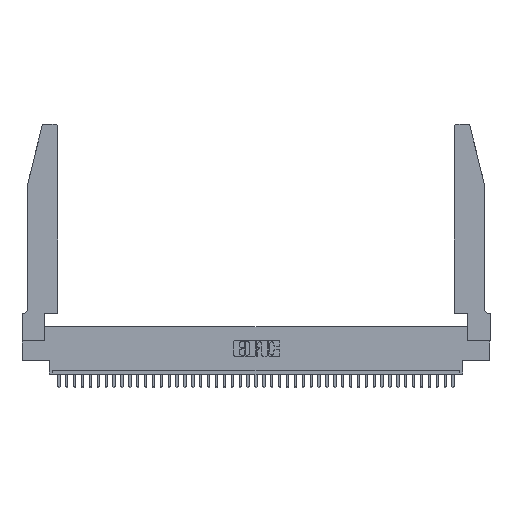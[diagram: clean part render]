
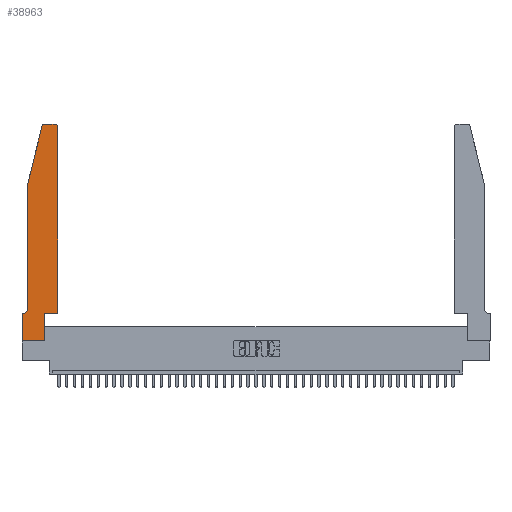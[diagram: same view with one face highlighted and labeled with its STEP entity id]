
A CAD part, top view. The second image highlights one B-rep face of the part: STEP entity #38963.
In plain terms, the highlighted planar face has unit normal (0, 0, 1).
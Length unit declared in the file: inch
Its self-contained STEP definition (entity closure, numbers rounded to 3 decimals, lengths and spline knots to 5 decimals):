
#378 = VECTOR ( 'NONE', #20610, 39.37008 ) ;
#417 = DIRECTION ( 'NONE',  ( 0., 0., 1. ) ) ;
#780 = VERTEX_POINT ( 'NONE', #36501 ) ;
#1311 = VERTEX_POINT ( 'NONE', #11483 ) ;
#1314 = VERTEX_POINT ( 'NONE', #11922 ) ;
#1644 = ORIENTED_EDGE ( 'NONE', *, *, #15194, .T. ) ;
#1787 = AXIS2_PLACEMENT_3D ( 'NONE', #8677, #15035, #21431 ) ;
#1841 = ORIENTED_EDGE ( 'NONE', *, *, #27327, .T. ) ;
#2714 = VECTOR ( 'NONE', #11933, 39.37008 ) ;
#3234 = VECTOR ( 'NONE', #31210, 39.37008 ) ;
#3577 = CIRCLE ( 'NONE', #1787, 0.07 ) ;
#3644 = LINE ( 'NONE', #36861, #30088 ) ;
#3887 = DIRECTION ( 'NONE',  ( 0., 0., 1. ) ) ;
#4013 = ORIENTED_EDGE ( 'NONE', *, *, #22150, .T. ) ;
#4426 = VERTEX_POINT ( 'NONE', #34378 ) ;
#4610 = DIRECTION ( 'NONE',  ( 0., -1., 0. ) ) ;
#5189 = CARTESIAN_POINT ( 'NONE',  ( 0.284, 2.72, 0.37 ) ) ;
#7242 = VERTEX_POINT ( 'NONE', #28314 ) ;
#7512 = CARTESIAN_POINT ( 'NONE',  ( 0.0755, 2., 0.37 ) ) ;
#8570 = ORIENTED_EDGE ( 'NONE', *, *, #21283, .T. ) ;
#8677 = CARTESIAN_POINT ( 'NONE',  ( 0.0055, 0.42, 0.37 ) ) ;
#8825 = VERTEX_POINT ( 'NONE', #28804 ) ;
#8885 = LINE ( 'NONE', #33943, #2714 ) ;
#9082 = AXIS2_PLACEMENT_3D ( 'NONE', #39704, #3887, #14320 ) ;
#9258 = DIRECTION ( 'NONE',  ( 0., 1., 0. ) ) ;
#10153 = VERTEX_POINT ( 'NONE', #36741 ) ;
#10204 = EDGE_LOOP ( 'NONE', ( #28763, #8570, #1841, #1644, #36367, #24538, #15567, #11738, #4013, #31337, #11991, #17164 ) ) ;
#10351 = AXIS2_PLACEMENT_3D ( 'NONE', #5189, #15029, #18297 ) ;
#10630 = VECTOR ( 'NONE', #33757, 39.37008 ) ;
#10833 = CARTESIAN_POINT ( 'NONE',  ( 0.0755, 2., 0.37 ) ) ;
#11483 = CARTESIAN_POINT ( 'NONE',  ( 0.4505, 0.35, 0.37 ) ) ;
#11738 = ORIENTED_EDGE ( 'NONE', *, *, #30949, .T. ) ;
#11922 = CARTESIAN_POINT ( 'NONE',  ( 0.2865, 0.35, 0.37 ) ) ;
#11933 = DIRECTION ( 'NONE',  ( 1., 0., 0. ) ) ;
#11991 = ORIENTED_EDGE ( 'NONE', *, *, #23770, .T. ) ;
#12405 = LINE ( 'NONE', #20170, #26552 ) ;
#13259 = LINE ( 'NONE', #35514, #36599 ) ;
#13588 = DIRECTION ( 'NONE',  ( 1., 0., 0. ) ) ;
#13979 = CARTESIAN_POINT ( 'NONE',  ( 0.4505, 0.35, 0.37 ) ) ;
#14320 = DIRECTION ( 'NONE',  ( 1., 0., 0. ) ) ;
#14397 = VERTEX_POINT ( 'NONE', #15028 ) ;
#15028 = CARTESIAN_POINT ( 'NONE',  ( 0., 0., 0.37 ) ) ;
#15029 = DIRECTION ( 'NONE',  ( 0., 0., 1. ) ) ;
#15035 = DIRECTION ( 'NONE',  ( 0., 0., -1. ) ) ;
#15194 = EDGE_CURVE ( 'NONE', #4426, #8825, #32980, .T. ) ;
#15567 = ORIENTED_EDGE ( 'NONE', *, *, #37715, .T. ) ;
#17164 = ORIENTED_EDGE ( 'NONE', *, *, #21461, .T. ) ;
#17493 = CARTESIAN_POINT ( 'NONE',  ( 0., 0.35, 0.37 ) ) ;
#18297 = DIRECTION ( 'NONE',  ( 1., 0., 0. ) ) ;
#18434 = EDGE_CURVE ( 'NONE', #1314, #1311, #32699, .T. ) ;
#18967 = VECTOR ( 'NONE', #9258, 39.37008 ) ;
#20148 = CARTESIAN_POINT ( 'NONE',  ( 0., 0.35, 0.37 ) ) ;
#20170 = CARTESIAN_POINT ( 'NONE',  ( 0.0755, 0.35, 0.37 ) ) ;
#20222 = FACE_OUTER_BOUND ( 'NONE', #10204, .T. ) ;
#20610 = DIRECTION ( 'NONE',  ( 0., -1., 0. ) ) ;
#21283 = EDGE_CURVE ( 'NONE', #32527, #7242, #30220, .T. ) ;
#21431 = DIRECTION ( 'NONE',  ( -1., 0., 0. ) ) ;
#21461 = EDGE_CURVE ( 'NONE', #37892, #27038, #41509, .T. ) ;
#22150 = EDGE_CURVE ( 'NONE', #780, #1314, #34272, .T. ) ;
#22789 = CARTESIAN_POINT ( 'NONE',  ( 0.4205, 2.75, 0.37 ) ) ;
#23664 = EDGE_CURVE ( 'NONE', #8825, #10153, #3577, .T. ) ;
#23770 = EDGE_CURVE ( 'NONE', #1311, #37892, #27543, .T. ) ;
#24412 = CARTESIAN_POINT ( 'NONE',  ( 0.4505, 2.72, 0.37 ) ) ;
#24538 = ORIENTED_EDGE ( 'NONE', *, *, #41795, .T. ) ;
#26020 = DIRECTION ( 'NONE',  ( 0., 1., 0. ) ) ;
#26186 = EDGE_CURVE ( 'NONE', #27038, #32527, #13259, .T. ) ;
#26319 = VERTEX_POINT ( 'NONE', #17493 ) ;
#26552 = VECTOR ( 'NONE', #33046, 39.37008 ) ;
#27038 = VERTEX_POINT ( 'NONE', #22789 ) ;
#27327 = EDGE_CURVE ( 'NONE', #7242, #4426, #40663, .T. ) ;
#27543 = LINE ( 'NONE', #34883, #18967 ) ;
#28314 = CARTESIAN_POINT ( 'NONE',  ( 0.25487, 2.72718, 0.37 ) ) ;
#28763 = ORIENTED_EDGE ( 'NONE', *, *, #26186, .T. ) ;
#28780 = VECTOR ( 'NONE', #26020, 39.37008 ) ;
#28804 = CARTESIAN_POINT ( 'NONE',  ( 0.0755, 0.42, 0.37 ) ) ;
#29298 = AXIS2_PLACEMENT_3D ( 'NONE', #20148, #417, #13588 ) ;
#30088 = VECTOR ( 'NONE', #4610, 39.37008 ) ;
#30220 = CIRCLE ( 'NONE', #10351, 0.03 ) ;
#30676 = DIRECTION ( 'NONE',  ( -1., 0., 0. ) ) ;
#30949 = EDGE_CURVE ( 'NONE', #14397, #780, #8885, .T. ) ;
#31210 = DIRECTION ( 'NONE',  ( 1., 0., 0. ) ) ;
#31337 = ORIENTED_EDGE ( 'NONE', *, *, #18434, .T. ) ;
#32527 = VERTEX_POINT ( 'NONE', #41782 ) ;
#32699 = LINE ( 'NONE', #13979, #3234 ) ;
#32980 = LINE ( 'NONE', #10833, #378 ) ;
#33046 = DIRECTION ( 'NONE',  ( -1., 0., 0. ) ) ;
#33757 = DIRECTION ( 'NONE',  ( -0.239, -0.971, 0. ) ) ;
#33943 = CARTESIAN_POINT ( 'NONE',  ( 0., 0., 0.37 ) ) ;
#34272 = LINE ( 'NONE', #35510, #28780 ) ;
#34378 = CARTESIAN_POINT ( 'NONE',  ( 0.0755, 2., 0.37 ) ) ;
#34883 = CARTESIAN_POINT ( 'NONE',  ( 0.4505, 0.35, 0.37 ) ) ;
#35510 = CARTESIAN_POINT ( 'NONE',  ( 0.2865, 0.35, 0.37 ) ) ;
#35514 = CARTESIAN_POINT ( 'NONE',  ( 0.2605, 2.75, 0.37 ) ) ;
#36158 = PLANE ( 'NONE',  #29298 ) ;
#36367 = ORIENTED_EDGE ( 'NONE', *, *, #23664, .T. ) ;
#36501 = CARTESIAN_POINT ( 'NONE',  ( 0.2865, 0., 0.37 ) ) ;
#36599 = VECTOR ( 'NONE', #30676, 39.37008 ) ;
#36741 = CARTESIAN_POINT ( 'NONE',  ( 0.0055, 0.35, 0.37 ) ) ;
#36861 = CARTESIAN_POINT ( 'NONE',  ( 0., 0., 0.37 ) ) ;
#37715 = EDGE_CURVE ( 'NONE', #26319, #14397, #3644, .T. ) ;
#37892 = VERTEX_POINT ( 'NONE', #24412 ) ;
#38963 = ADVANCED_FACE ( 'NONE', ( #20222 ), #36158, .T. ) ;
#39704 = CARTESIAN_POINT ( 'NONE',  ( 0.4205, 2.72, 0.37 ) ) ;
#40663 = LINE ( 'NONE', #7512, #10630 ) ;
#41509 = CIRCLE ( 'NONE', #9082, 0.03 ) ;
#41782 = CARTESIAN_POINT ( 'NONE',  ( 0.284, 2.75, 0.37 ) ) ;
#41795 = EDGE_CURVE ( 'NONE', #10153, #26319, #12405, .T. ) ;
